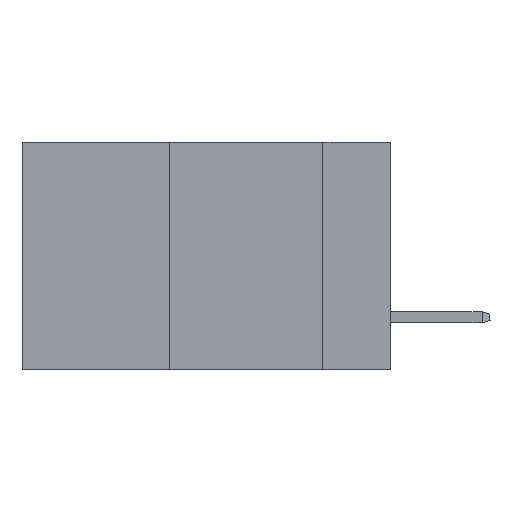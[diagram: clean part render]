
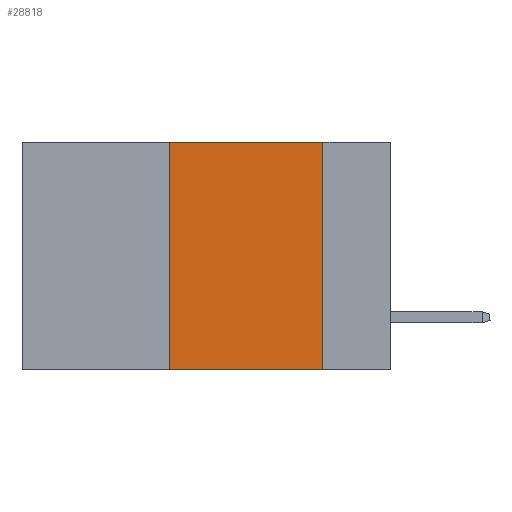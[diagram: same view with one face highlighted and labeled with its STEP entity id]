
A CAD part, left-side view. The second image highlights one B-rep face of the part: STEP entity #28818.
In plain terms, the highlighted planar face has unit normal (-1, 0, 0).
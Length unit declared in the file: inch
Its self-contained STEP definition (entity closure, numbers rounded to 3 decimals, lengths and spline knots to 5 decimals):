
#397 = DIRECTION ( 'NONE',  ( 0., 0., -1. ) ) ;
#3354 = LINE ( 'NONE', #6163, #40672 ) ;
#3606 = LINE ( 'NONE', #34592, #19933 ) ;
#5664 = VERTEX_POINT ( 'NONE', #39165 ) ;
#6163 = CARTESIAN_POINT ( 'NONE',  ( 0., 0.6, 0. ) ) ;
#9794 = CARTESIAN_POINT ( 'NONE',  ( 0., 0.6, -0.37 ) ) ;
#10016 = DIRECTION ( 'NONE',  ( 1., 0., 0. ) ) ;
#10963 = CARTESIAN_POINT ( 'NONE',  ( 0., 0.36, 0. ) ) ;
#14292 = EDGE_CURVE ( 'NONE', #29327, #29746, #24585, .T. ) ;
#14386 = CARTESIAN_POINT ( 'NONE',  ( 0., 0.11, -0.37 ) ) ;
#15150 = EDGE_LOOP ( 'NONE', ( #27591, #18469, #31319, #17812 ) ) ;
#17540 = VECTOR ( 'NONE', #19356, 39.37008 ) ;
#17746 = EDGE_CURVE ( 'NONE', #5664, #39874, #3606, .T. ) ;
#17812 = ORIENTED_EDGE ( 'NONE', *, *, #22080, .T. ) ;
#18469 = ORIENTED_EDGE ( 'NONE', *, *, #20021, .F. ) ;
#19356 = DIRECTION ( 'NONE',  ( 0., -1., 0. ) ) ;
#19418 = CARTESIAN_POINT ( 'NONE',  ( 0., 0.11, 0. ) ) ;
#19933 = VECTOR ( 'NONE', #38726, 39.37008 ) ;
#20021 = EDGE_CURVE ( 'NONE', #39874, #29327, #3354, .T. ) ;
#20483 = VECTOR ( 'NONE', #397, 39.37008 ) ;
#22017 = DIRECTION ( 'NONE',  ( 0., -1., 0. ) ) ;
#22080 = EDGE_CURVE ( 'NONE', #5664, #29746, #34944, .T. ) ;
#24585 = LINE ( 'NONE', #29675, #20483 ) ;
#26409 = DIRECTION ( 'NONE',  ( 0., 0., -1. ) ) ;
#27591 = ORIENTED_EDGE ( 'NONE', *, *, #14292, .F. ) ;
#28818 = ADVANCED_FACE ( 'NONE', ( #38073 ), #29306, .F. ) ;
#29306 = PLANE ( 'NONE',  #42184 ) ;
#29327 = VERTEX_POINT ( 'NONE', #19418 ) ;
#29675 = CARTESIAN_POINT ( 'NONE',  ( 0., 0.11, 0. ) ) ;
#29746 = VERTEX_POINT ( 'NONE', #14386 ) ;
#31319 = ORIENTED_EDGE ( 'NONE', *, *, #17746, .F. ) ;
#34592 = CARTESIAN_POINT ( 'NONE',  ( 0., 0.36, 0. ) ) ;
#34944 = LINE ( 'NONE', #9794, #17540 ) ;
#38073 = FACE_OUTER_BOUND ( 'NONE', #15150, .T. ) ;
#38726 = DIRECTION ( 'NONE',  ( 0., 0., 1. ) ) ;
#39165 = CARTESIAN_POINT ( 'NONE',  ( 0., 0.36, -0.37 ) ) ;
#39874 = VERTEX_POINT ( 'NONE', #10963 ) ;
#40672 = VECTOR ( 'NONE', #22017, 39.37008 ) ;
#42184 = AXIS2_PLACEMENT_3D ( 'NONE', #42324, #10016, #26409 ) ;
#42324 = CARTESIAN_POINT ( 'NONE',  ( 0., 0.6, 0. ) ) ;
